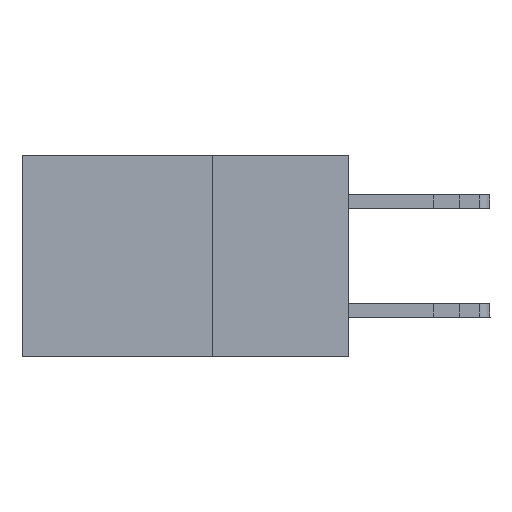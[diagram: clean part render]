
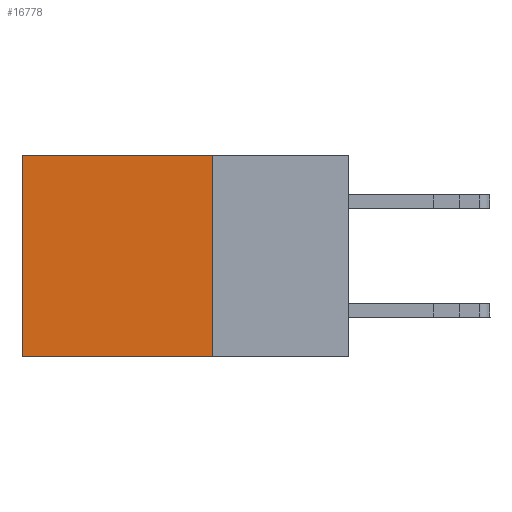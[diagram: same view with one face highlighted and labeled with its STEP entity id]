
A CAD part, left-side view. The second image highlights one B-rep face of the part: STEP entity #16778.
In plain terms, the highlighted planar face has unit normal (-1, 0, 0).
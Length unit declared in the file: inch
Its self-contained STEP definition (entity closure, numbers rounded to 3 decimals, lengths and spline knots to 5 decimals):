
#682 = FACE_OUTER_BOUND ( 'NONE', #19479, .T. ) ;
#847 = DIRECTION ( 'NONE',  ( 0., 1., 0. ) ) ;
#1126 = ORIENTED_EDGE ( 'NONE', *, *, #5282, .F. ) ;
#3438 = DIRECTION ( 'NONE',  ( 1., 0., 0. ) ) ;
#4176 = ORIENTED_EDGE ( 'NONE', *, *, #22785, .T. ) ;
#4903 = DIRECTION ( 'NONE',  ( 0., 1., 0. ) ) ;
#4990 = LINE ( 'NONE', #20953, #19766 ) ;
#5282 = EDGE_CURVE ( 'NONE', #11889, #11584, #10992, .T. ) ;
#6335 = VERTEX_POINT ( 'NONE', #11580 ) ;
#6453 = EDGE_CURVE ( 'NONE', #16453, #6335, #10369, .T. ) ;
#6678 = AXIS2_PLACEMENT_3D ( 'NONE', #9018, #3438, #7307 ) ;
#7307 = DIRECTION ( 'NONE',  ( 0., 0., -1. ) ) ;
#7911 = DIRECTION ( 'NONE',  ( 0., 0., -1. ) ) ;
#8522 = LINE ( 'NONE', #23550, #17237 ) ;
#8926 = DIRECTION ( 'NONE',  ( 0., 0., -1. ) ) ;
#9018 = CARTESIAN_POINT ( 'NONE',  ( 0.298, 0.25, 0. ) ) ;
#10369 = LINE ( 'NONE', #19432, #14408 ) ;
#10704 = VECTOR ( 'NONE', #4903, 39.37008 ) ;
#10949 = PLANE ( 'NONE',  #6678 ) ;
#10992 = LINE ( 'NONE', #23409, #10704 ) ;
#11523 = EDGE_CURVE ( 'NONE', #16453, #11889, #4990, .T. ) ;
#11580 = CARTESIAN_POINT ( 'NONE',  ( 0.298, 0.6, 0. ) ) ;
#11584 = VERTEX_POINT ( 'NONE', #22848 ) ;
#11889 = VERTEX_POINT ( 'NONE', #11979 ) ;
#11979 = CARTESIAN_POINT ( 'NONE',  ( 0.298, 0.25, -0.37 ) ) ;
#12916 = ORIENTED_EDGE ( 'NONE', *, *, #6453, .T. ) ;
#14408 = VECTOR ( 'NONE', #847, 39.37008 ) ;
#16354 = CARTESIAN_POINT ( 'NONE',  ( 0.298, 0.25, 0. ) ) ;
#16453 = VERTEX_POINT ( 'NONE', #16354 ) ;
#16778 = ADVANCED_FACE ( 'NONE', ( #682 ), #10949, .F. ) ;
#17237 = VECTOR ( 'NONE', #8926, 39.37008 ) ;
#19432 = CARTESIAN_POINT ( 'NONE',  ( 0.298, 0.25, 0. ) ) ;
#19479 = EDGE_LOOP ( 'NONE', ( #4176, #1126, #22805, #12916 ) ) ;
#19766 = VECTOR ( 'NONE', #7911, 39.37008 ) ;
#20953 = CARTESIAN_POINT ( 'NONE',  ( 0.298, 0.25, 0. ) ) ;
#22785 = EDGE_CURVE ( 'NONE', #6335, #11584, #8522, .T. ) ;
#22805 = ORIENTED_EDGE ( 'NONE', *, *, #11523, .F. ) ;
#22848 = CARTESIAN_POINT ( 'NONE',  ( 0.298, 0.6, -0.37 ) ) ;
#23409 = CARTESIAN_POINT ( 'NONE',  ( 0.298, 0.25, -0.37 ) ) ;
#23550 = CARTESIAN_POINT ( 'NONE',  ( 0.298, 0.6, 0. ) ) ;
